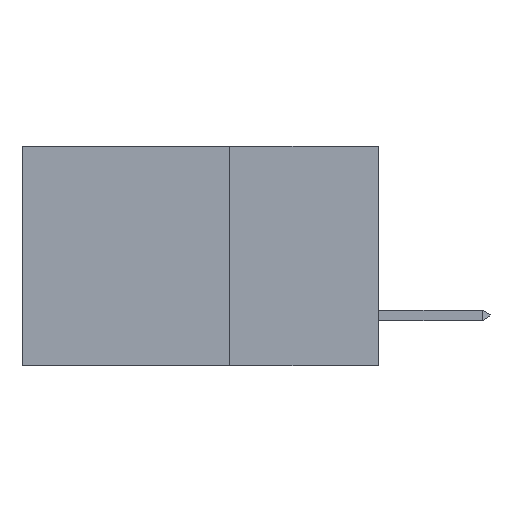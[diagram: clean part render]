
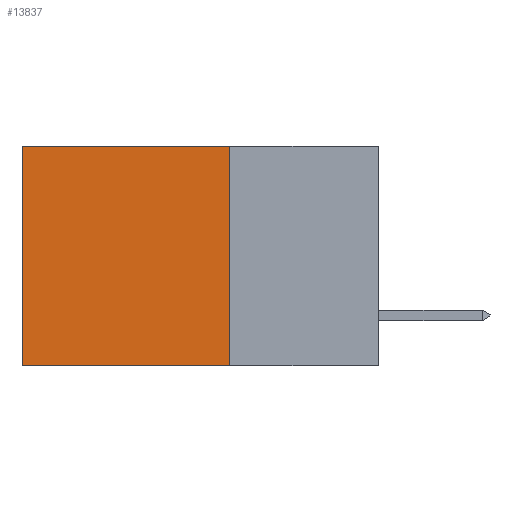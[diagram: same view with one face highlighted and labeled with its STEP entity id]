
A CAD part, left-side view. The second image highlights one B-rep face of the part: STEP entity #13837.
In plain terms, the highlighted planar face has unit normal (-1, 0, 0).
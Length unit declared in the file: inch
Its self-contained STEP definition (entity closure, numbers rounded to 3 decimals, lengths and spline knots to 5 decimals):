
#8 = ORIENTED_EDGE ( 'NONE', *, *, #1818, .F. ) ;
#759 = FACE_OUTER_BOUND ( 'NONE', #4688, .T. ) ;
#782 = CARTESIAN_POINT ( 'NONE',  ( 0.2615, 0.6, -0.37 ) ) ;
#954 = EDGE_CURVE ( 'NONE', #7403, #5593, #4200, .T. ) ;
#1581 = VECTOR ( 'NONE', #7672, 39.37008 ) ;
#1818 = EDGE_CURVE ( 'NONE', #1930, #7403, #10634, .T. ) ;
#1930 = VERTEX_POINT ( 'NONE', #13794 ) ;
#2778 = DIRECTION ( 'NONE',  ( 0., 0., -1. ) ) ;
#3170 = CARTESIAN_POINT ( 'NONE',  ( 0.2615, 0.25, 0. ) ) ;
#3277 = LINE ( 'NONE', #4164, #5624 ) ;
#3441 = DIRECTION ( 'NONE',  ( 1., 0., 0. ) ) ;
#4062 = EDGE_CURVE ( 'NONE', #10627, #5593, #3277, .T. ) ;
#4093 = CARTESIAN_POINT ( 'NONE',  ( 0.2615, 0.25, -0.37 ) ) ;
#4164 = CARTESIAN_POINT ( 'NONE',  ( 0.2615, 0.6, -0.37 ) ) ;
#4200 = LINE ( 'NONE', #4093, #14296 ) ;
#4212 = DIRECTION ( 'NONE',  ( 0., 0., -1. ) ) ;
#4440 = PLANE ( 'NONE',  #4698 ) ;
#4637 = DIRECTION ( 'NONE',  ( 0., 0., -1. ) ) ;
#4688 = EDGE_LOOP ( 'NONE', ( #5187, #14799, #8, #5336 ) ) ;
#4698 = AXIS2_PLACEMENT_3D ( 'NONE', #14824, #3441, #4637 ) ;
#4834 = LINE ( 'NONE', #3170, #1581 ) ;
#5187 = ORIENTED_EDGE ( 'NONE', *, *, #4062, .T. ) ;
#5336 = ORIENTED_EDGE ( 'NONE', *, *, #9996, .T. ) ;
#5377 = CARTESIAN_POINT ( 'NONE',  ( 0.2615, 0.6, 0. ) ) ;
#5593 = VERTEX_POINT ( 'NONE', #782 ) ;
#5624 = VECTOR ( 'NONE', #4212, 39.37008 ) ;
#5972 = VECTOR ( 'NONE', #2778, 39.37008 ) ;
#7403 = VERTEX_POINT ( 'NONE', #11199 ) ;
#7672 = DIRECTION ( 'NONE',  ( 0., 1., 0. ) ) ;
#8750 = DIRECTION ( 'NONE',  ( 0., 1., 0. ) ) ;
#9996 = EDGE_CURVE ( 'NONE', #1930, #10627, #4834, .T. ) ;
#10627 = VERTEX_POINT ( 'NONE', #5377 ) ;
#10634 = LINE ( 'NONE', #14204, #5972 ) ;
#11199 = CARTESIAN_POINT ( 'NONE',  ( 0.2615, 0.25, -0.37 ) ) ;
#13794 = CARTESIAN_POINT ( 'NONE',  ( 0.2615, 0.25, 0. ) ) ;
#13837 = ADVANCED_FACE ( 'NONE', ( #759 ), #4440, .F. ) ;
#14204 = CARTESIAN_POINT ( 'NONE',  ( 0.2615, 0.25, -0.37 ) ) ;
#14296 = VECTOR ( 'NONE', #8750, 39.37008 ) ;
#14799 = ORIENTED_EDGE ( 'NONE', *, *, #954, .F. ) ;
#14824 = CARTESIAN_POINT ( 'NONE',  ( 0.2615, 0.25, -0.37 ) ) ;
